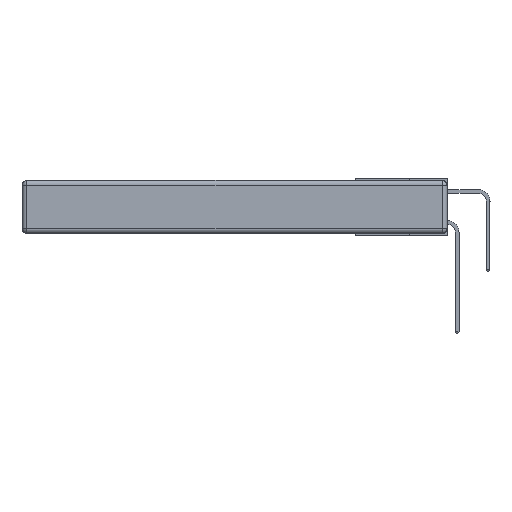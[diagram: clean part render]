
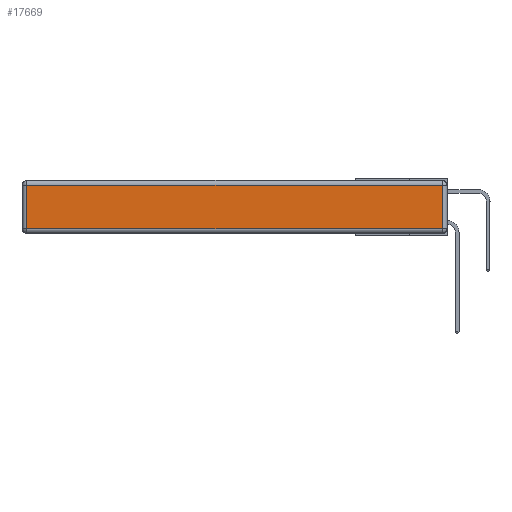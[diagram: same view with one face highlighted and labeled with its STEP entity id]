
A CAD part, left-side view. The second image highlights one B-rep face of the part: STEP entity #17669.
In plain terms, the highlighted planar face has unit normal (-1, 0, 0).
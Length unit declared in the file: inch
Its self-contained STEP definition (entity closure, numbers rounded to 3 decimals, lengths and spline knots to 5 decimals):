
#234 = PLANE ( 'NONE',  #11951 ) ;
#920 = VERTEX_POINT ( 'NONE', #17401 ) ;
#922 = EDGE_CURVE ( 'NONE', #3693, #18081, #16385, .T. ) ;
#1379 = VECTOR ( 'NONE', #20681, 39.37008 ) ;
#2010 = CARTESIAN_POINT ( 'NONE',  ( 0., 0., -0.343 ) ) ;
#2833 = EDGE_CURVE ( 'NONE', #18081, #9656, #18742, .T. ) ;
#3570 = LINE ( 'NONE', #10137, #22368 ) ;
#3693 = VERTEX_POINT ( 'NONE', #14650 ) ;
#3944 = ORIENTED_EDGE ( 'NONE', *, *, #6819, .T. ) ;
#5421 = CARTESIAN_POINT ( 'NONE',  ( 0., 0., -0.313 ) ) ;
#5942 = FACE_OUTER_BOUND ( 'NONE', #17027, .T. ) ;
#6429 = ORIENTED_EDGE ( 'NONE', *, *, #20707, .T. ) ;
#6819 = EDGE_CURVE ( 'NONE', #9656, #920, #3570, .T. ) ;
#7977 = VECTOR ( 'NONE', #16132, 39.37008 ) ;
#8792 = VECTOR ( 'NONE', #11648, 39.37008 ) ;
#8864 = ORIENTED_EDGE ( 'NONE', *, *, #922, .T. ) ;
#9103 = DIRECTION ( 'NONE',  ( -1., 0., 0. ) ) ;
#9656 = VERTEX_POINT ( 'NONE', #11455 ) ;
#10137 = CARTESIAN_POINT ( 'NONE',  ( 0., 2.72, -0.343 ) ) ;
#11455 = CARTESIAN_POINT ( 'NONE',  ( 0., 2.72, -0.03 ) ) ;
#11648 = DIRECTION ( 'NONE',  ( 0., 1., 0. ) ) ;
#11951 = AXIS2_PLACEMENT_3D ( 'NONE', #2010, #9103, #14296 ) ;
#13245 = LINE ( 'NONE', #5421, #7977 ) ;
#13445 = CARTESIAN_POINT ( 'NONE',  ( 0., 2.75, -0.03 ) ) ;
#14296 = DIRECTION ( 'NONE',  ( 0., 0., 1. ) ) ;
#14311 = CARTESIAN_POINT ( 'NONE',  ( 0., 0.03, -0.03 ) ) ;
#14650 = CARTESIAN_POINT ( 'NONE',  ( 0., 0.03, -0.313 ) ) ;
#15315 = ORIENTED_EDGE ( 'NONE', *, *, #2833, .T. ) ;
#15800 = CARTESIAN_POINT ( 'NONE',  ( 0., 0.03, -0.343 ) ) ;
#16132 = DIRECTION ( 'NONE',  ( 0., -1., 0. ) ) ;
#16385 = LINE ( 'NONE', #15800, #1379 ) ;
#17027 = EDGE_LOOP ( 'NONE', ( #6429, #8864, #15315, #3944 ) ) ;
#17401 = CARTESIAN_POINT ( 'NONE',  ( 0., 2.72, -0.313 ) ) ;
#17669 = ADVANCED_FACE ( 'NONE', ( #5942 ), #234, .T. ) ;
#18081 = VERTEX_POINT ( 'NONE', #14311 ) ;
#18742 = LINE ( 'NONE', #13445, #8792 ) ;
#18999 = DIRECTION ( 'NONE',  ( 0., 0., -1. ) ) ;
#20681 = DIRECTION ( 'NONE',  ( 0., 0., 1. ) ) ;
#20707 = EDGE_CURVE ( 'NONE', #920, #3693, #13245, .T. ) ;
#22368 = VECTOR ( 'NONE', #18999, 39.37008 ) ;
